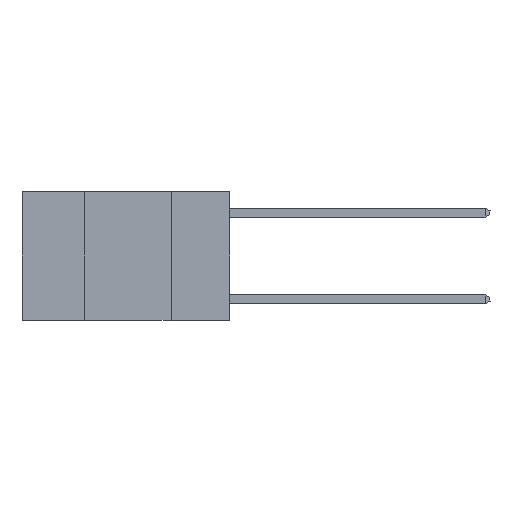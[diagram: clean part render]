
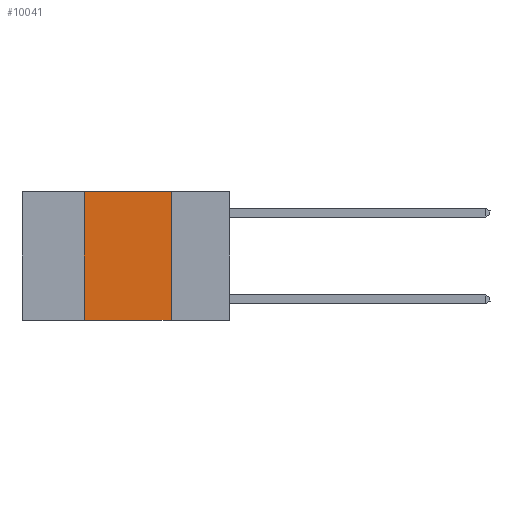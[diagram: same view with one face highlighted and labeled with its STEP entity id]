
A CAD part, left-side view. The second image highlights one B-rep face of the part: STEP entity #10041.
In plain terms, the highlighted planar face has unit normal (-1, 0, 0).
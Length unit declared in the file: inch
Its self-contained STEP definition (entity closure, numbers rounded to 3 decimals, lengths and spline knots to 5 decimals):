
#442 = ORIENTED_EDGE ( 'NONE', *, *, #14489, .F. ) ;
#549 = DIRECTION ( 'NONE',  ( 0., 0., 1. ) ) ;
#1237 = EDGE_CURVE ( 'NONE', #18860, #18677, #14932, .T. ) ;
#1328 = CARTESIAN_POINT ( 'NONE',  ( 0., 0.17, 0. ) ) ;
#2408 = EDGE_LOOP ( 'NONE', ( #17481, #4458, #442, #9512 ) ) ;
#3183 = CARTESIAN_POINT ( 'NONE',  ( 0., 0.17, -0.37 ) ) ;
#3972 = DIRECTION ( 'NONE',  ( 1., 0., 0. ) ) ;
#4458 = ORIENTED_EDGE ( 'NONE', *, *, #1237, .F. ) ;
#4735 = DIRECTION ( 'NONE',  ( 0., 0., -1. ) ) ;
#4937 = CARTESIAN_POINT ( 'NONE',  ( 0., 0.42, -0.37 ) ) ;
#5486 = VERTEX_POINT ( 'NONE', #4937 ) ;
#8030 = LINE ( 'NONE', #1328, #21046 ) ;
#9512 = ORIENTED_EDGE ( 'NONE', *, *, #12360, .T. ) ;
#10041 = ADVANCED_FACE ( 'NONE', ( #15750 ), #10762, .F. ) ;
#10375 = VECTOR ( 'NONE', #16892, 39.37008 ) ;
#10472 = DIRECTION ( 'NONE',  ( 0., -1., 0. ) ) ;
#10762 = PLANE ( 'NONE',  #12661 ) ;
#11657 = LINE ( 'NONE', #18933, #16718 ) ;
#12360 = EDGE_CURVE ( 'NONE', #5486, #20308, #11657, .T. ) ;
#12482 = CARTESIAN_POINT ( 'NONE',  ( 0., 0.42, 0. ) ) ;
#12661 = AXIS2_PLACEMENT_3D ( 'NONE', #14201, #3972, #15890 ) ;
#13255 = CARTESIAN_POINT ( 'NONE',  ( 0., 0.42, 0. ) ) ;
#13500 = CARTESIAN_POINT ( 'NONE',  ( 0., 0.6, 0. ) ) ;
#14201 = CARTESIAN_POINT ( 'NONE',  ( 0., 0.6, 0. ) ) ;
#14489 = EDGE_CURVE ( 'NONE', #5486, #18860, #16475, .T. ) ;
#14932 = LINE ( 'NONE', #13500, #10375 ) ;
#15750 = FACE_OUTER_BOUND ( 'NONE', #2408, .T. ) ;
#15835 = CARTESIAN_POINT ( 'NONE',  ( 0., 0.17, 0. ) ) ;
#15890 = DIRECTION ( 'NONE',  ( 0., 0., -1. ) ) ;
#16475 = LINE ( 'NONE', #12482, #17515 ) ;
#16718 = VECTOR ( 'NONE', #10472, 39.37008 ) ;
#16892 = DIRECTION ( 'NONE',  ( 0., -1., 0. ) ) ;
#17481 = ORIENTED_EDGE ( 'NONE', *, *, #18847, .F. ) ;
#17515 = VECTOR ( 'NONE', #549, 39.37008 ) ;
#18677 = VERTEX_POINT ( 'NONE', #15835 ) ;
#18847 = EDGE_CURVE ( 'NONE', #18677, #20308, #8030, .T. ) ;
#18860 = VERTEX_POINT ( 'NONE', #13255 ) ;
#18933 = CARTESIAN_POINT ( 'NONE',  ( 0., 0.6, -0.37 ) ) ;
#20308 = VERTEX_POINT ( 'NONE', #3183 ) ;
#21046 = VECTOR ( 'NONE', #4735, 39.37008 ) ;
